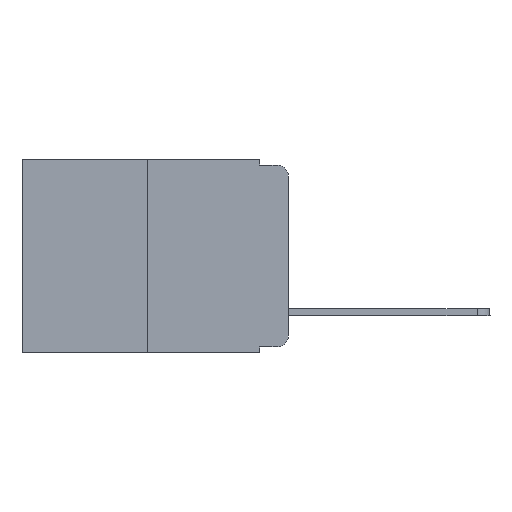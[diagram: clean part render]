
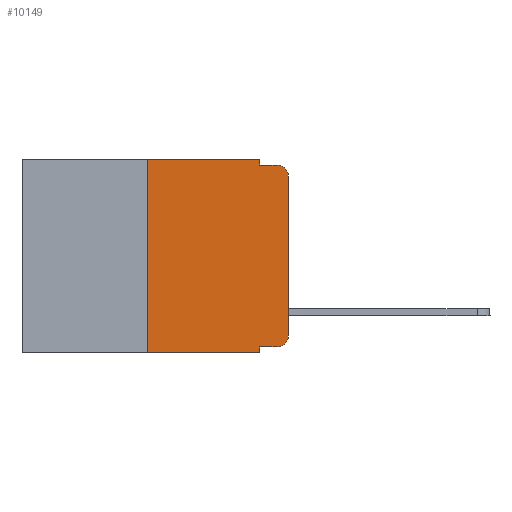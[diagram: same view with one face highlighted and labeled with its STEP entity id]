
A CAD part, left-side view. The second image highlights one B-rep face of the part: STEP entity #10149.
In plain terms, the highlighted planar face has unit normal (-1, 0, 0).
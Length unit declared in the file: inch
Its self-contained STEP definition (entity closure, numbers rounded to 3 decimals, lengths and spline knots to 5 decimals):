
#161 = AXIS2_PLACEMENT_3D ( 'NONE', #1748, #4748, #10141 ) ;
#163 = VECTOR ( 'NONE', #10640, 39.37008 ) ;
#184 = EDGE_CURVE ( 'NONE', #7810, #3105, #2323, .T. ) ;
#241 = CARTESIAN_POINT ( 'NONE',  ( 0., 0.051, 0. ) ) ;
#355 = CARTESIAN_POINT ( 'NONE',  ( 0., 0.051, 0. ) ) ;
#534 = CARTESIAN_POINT ( 'NONE',  ( 0., 0.25, -0.343 ) ) ;
#577 = EDGE_CURVE ( 'NONE', #10648, #3750, #9570, .T. ) ;
#607 = FACE_OUTER_BOUND ( 'NONE', #9200, .T. ) ;
#670 = ORIENTED_EDGE ( 'NONE', *, *, #7809, .F. ) ;
#999 = EDGE_CURVE ( 'NONE', #3750, #1130, #9054, .T. ) ;
#1077 = VECTOR ( 'NONE', #8115, 39.37008 ) ;
#1130 = VERTEX_POINT ( 'NONE', #6806 ) ;
#1458 = ORIENTED_EDGE ( 'NONE', *, *, #8495, .F. ) ;
#1748 = CARTESIAN_POINT ( 'NONE',  ( 0., 0.02, -0.03 ) ) ;
#1767 = ORIENTED_EDGE ( 'NONE', *, *, #6593, .T. ) ;
#1781 = CARTESIAN_POINT ( 'NONE',  ( 0., 0.051, -0.01 ) ) ;
#2213 = EDGE_CURVE ( 'NONE', #4562, #7717, #3240, .T. ) ;
#2323 = LINE ( 'NONE', #6477, #7240 ) ;
#2671 = CARTESIAN_POINT ( 'NONE',  ( 0., 0.02, -0.313 ) ) ;
#2772 = DIRECTION ( 'NONE',  ( 0., 0., -1. ) ) ;
#2971 = LINE ( 'NONE', #6241, #163 ) ;
#3105 = VERTEX_POINT ( 'NONE', #241 ) ;
#3240 = LINE ( 'NONE', #1781, #1077 ) ;
#3302 = ORIENTED_EDGE ( 'NONE', *, *, #8001, .F. ) ;
#3307 = DIRECTION ( 'NONE',  ( 0., -1., 0. ) ) ;
#3437 = DIRECTION ( 'NONE',  ( 0., 0., -1. ) ) ;
#3506 = AXIS2_PLACEMENT_3D ( 'NONE', #2671, #13535, #11536 ) ;
#3750 = VERTEX_POINT ( 'NONE', #8636 ) ;
#3796 = CARTESIAN_POINT ( 'NONE',  ( 0., 0.25, 0. ) ) ;
#3942 = CARTESIAN_POINT ( 'NONE',  ( 0., 0.051, -0.333 ) ) ;
#4382 = PLANE ( 'NONE',  #13184 ) ;
#4562 = VERTEX_POINT ( 'NONE', #10388 ) ;
#4589 = VECTOR ( 'NONE', #9827, 39.37008 ) ;
#4748 = DIRECTION ( 'NONE',  ( -1., 0., 0. ) ) ;
#4933 = ORIENTED_EDGE ( 'NONE', *, *, #2213, .F. ) ;
#5471 = DIRECTION ( 'NONE',  ( 1., 0., 0. ) ) ;
#5490 = CARTESIAN_POINT ( 'NONE',  ( 0., 0.051, -0.333 ) ) ;
#5678 = VERTEX_POINT ( 'NONE', #8163 ) ;
#6131 = ORIENTED_EDGE ( 'NONE', *, *, #999, .T. ) ;
#6219 = DIRECTION ( 'NONE',  ( 0., -1., 0. ) ) ;
#6241 = CARTESIAN_POINT ( 'NONE',  ( 0., 0.25, 0. ) ) ;
#6477 = CARTESIAN_POINT ( 'NONE',  ( 0., 0.473, 0. ) ) ;
#6576 = CARTESIAN_POINT ( 'NONE',  ( 0., 0.473, -0.343 ) ) ;
#6593 = EDGE_CURVE ( 'NONE', #1130, #13180, #10087, .T. ) ;
#6723 = CARTESIAN_POINT ( 'NONE',  ( 0., 0.02, -0.01 ) ) ;
#6806 = CARTESIAN_POINT ( 'NONE',  ( 0., 0., -0.313 ) ) ;
#7240 = VECTOR ( 'NONE', #12978, 39.37008 ) ;
#7717 = VERTEX_POINT ( 'NONE', #6723 ) ;
#7809 = EDGE_CURVE ( 'NONE', #3105, #4562, #9409, .T. ) ;
#7810 = VERTEX_POINT ( 'NONE', #3796 ) ;
#7819 = VECTOR ( 'NONE', #3307, 39.37008 ) ;
#8001 = EDGE_CURVE ( 'NONE', #13124, #7810, #2971, .T. ) ;
#8115 = DIRECTION ( 'NONE',  ( 0., -1., 0. ) ) ;
#8163 = CARTESIAN_POINT ( 'NONE',  ( 0., 0.051, -0.343 ) ) ;
#8438 = VECTOR ( 'NONE', #10258, 39.37008 ) ;
#8495 = EDGE_CURVE ( 'NONE', #10648, #5678, #11212, .T. ) ;
#8636 = CARTESIAN_POINT ( 'NONE',  ( 0., 0.02, -0.333 ) ) ;
#8766 = VECTOR ( 'NONE', #2772, 39.37008 ) ;
#8847 = CARTESIAN_POINT ( 'NONE',  ( 0., 0., -0.03 ) ) ;
#9054 = CIRCLE ( 'NONE', #3506, 0.02 ) ;
#9070 = CARTESIAN_POINT ( 'NONE',  ( 0., 0.051, 0. ) ) ;
#9086 = EDGE_CURVE ( 'NONE', #13180, #7717, #11049, .T. ) ;
#9115 = LINE ( 'NONE', #6576, #7819 ) ;
#9200 = EDGE_LOOP ( 'NONE', ( #1767, #13110, #4933, #670, #11305, #3302, #9985, #1458, #12753, #6131 ) ) ;
#9409 = LINE ( 'NONE', #9070, #8766 ) ;
#9570 = LINE ( 'NONE', #3942, #11227 ) ;
#9827 = DIRECTION ( 'NONE',  ( 0., 0., -1. ) ) ;
#9985 = ORIENTED_EDGE ( 'NONE', *, *, #12998, .T. ) ;
#10087 = LINE ( 'NONE', #13330, #8438 ) ;
#10141 = DIRECTION ( 'NONE',  ( 0., 0., -1. ) ) ;
#10149 = ADVANCED_FACE ( 'NONE', ( #607 ), #4382, .F. ) ;
#10258 = DIRECTION ( 'NONE',  ( 0., 0., 1. ) ) ;
#10388 = CARTESIAN_POINT ( 'NONE',  ( 0., 0.051, -0.01 ) ) ;
#10640 = DIRECTION ( 'NONE',  ( 0., 0., 1. ) ) ;
#10648 = VERTEX_POINT ( 'NONE', #5490 ) ;
#11049 = CIRCLE ( 'NONE', #161, 0.02 ) ;
#11212 = LINE ( 'NONE', #355, #4589 ) ;
#11227 = VECTOR ( 'NONE', #6219, 39.37008 ) ;
#11305 = ORIENTED_EDGE ( 'NONE', *, *, #184, .F. ) ;
#11536 = DIRECTION ( 'NONE',  ( 0., 0., -1. ) ) ;
#11796 = CARTESIAN_POINT ( 'NONE',  ( 0., 0.473, 0. ) ) ;
#12753 = ORIENTED_EDGE ( 'NONE', *, *, #577, .T. ) ;
#12978 = DIRECTION ( 'NONE',  ( 0., -1., 0. ) ) ;
#12998 = EDGE_CURVE ( 'NONE', #13124, #5678, #9115, .T. ) ;
#13110 = ORIENTED_EDGE ( 'NONE', *, *, #9086, .T. ) ;
#13124 = VERTEX_POINT ( 'NONE', #534 ) ;
#13180 = VERTEX_POINT ( 'NONE', #8847 ) ;
#13184 = AXIS2_PLACEMENT_3D ( 'NONE', #11796, #5471, #3437 ) ;
#13330 = CARTESIAN_POINT ( 'NONE',  ( 0., 0., 0. ) ) ;
#13535 = DIRECTION ( 'NONE',  ( -1., 0., 0. ) ) ;
